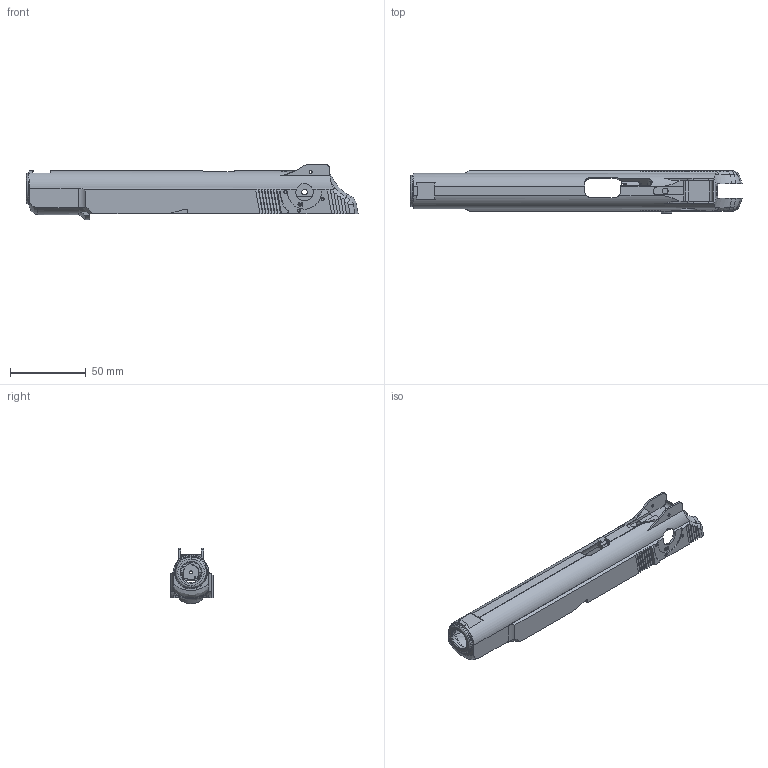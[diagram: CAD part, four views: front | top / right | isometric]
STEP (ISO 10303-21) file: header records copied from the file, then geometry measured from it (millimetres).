
FILE_DESCRIPTION(/* description */ (''),/* implementation_level */ '2;1');
FILE_NAME(/* name */ 'slide',/* time_stamp */ '2025-05-19T03:25:06+03:00',/* author */ (''),/* organization */ (''),/* preprocessor_version */ 'ST-DEVELOPER v16.5',/* originating_system */ '',/* authorisation */ '');
FILE_SCHEMA (('CONFIG_CONTROL_DESIGN'));
Length unit declared in the file: millimetre
Products named in the file (1): Document
Bounding box: 218.85 x 27.94 x 36.72 mm (x, y, z)
Volume: 38922.6 mm3; surface area: 34576.9 mm2
Topology: 1 solids, 1 shells, 439 faces, 1252 edges, 818 vertices
Faces by surface type: plane 322, cylinder 62, bspline 55
Entity records: 14755 total; most frequent: CARTESIAN_POINT 6474, ORIENTED_EDGE 2504, EDGE_CURVE 1252, B_SPLINE_CURVE_WITH_KNOTS 1095, VERTEX_POINT 818, EDGE_LOOP 460, ADVANCED_FACE 439, FACE_OUTER_BOUND 439
